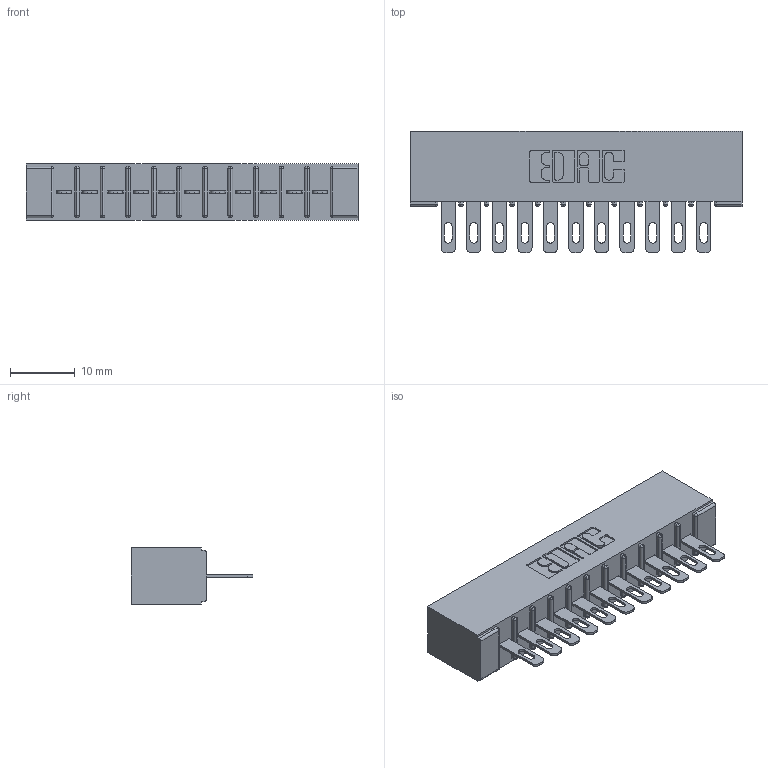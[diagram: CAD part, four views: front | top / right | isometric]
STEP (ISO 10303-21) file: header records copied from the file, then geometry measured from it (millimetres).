
FILE_DESCRIPTION (( 'STEP AP203' ), '1' );
FILE_NAME ('316-011-500-101.STEP', '2018-07-31T00:12:42', ( '' ), ( '' ), 'SwSTEP 2.0', 'SolidWorks 2016', '' );
FILE_SCHEMA (( 'CONFIG_CONTROL_DESIGN' ));
Length unit declared in the file: inch
Products named in the file (3): 306 Part_No Mounting; 306-290-001_100; 316-011-500-101
Assembly tree (12 placements, depth 2):
  316-011-500-101
    306 Part_No Mounting
    306-290-001_100  x11
Bounding box: 51.46 x 18.87 x 8.71 mm (x, y, z)
Volume: 3787 mm3; surface area: 5676.7 mm2
Topology: 12 solids, 12 shells, 944 faces, 2657 edges, 1710 vertices
Faces by surface type: plane 614, cylinder 286, sphere 44
Entity records: 14160 total; most frequent: CARTESIAN_POINT 2372, ORIENTED_EDGE 2346, DIRECTION 2343, EDGE_CURVE 1173, LINE 901, VECTOR 901, VERTEX_POINT 750, AXIS2_PLACEMENT_3D 721
